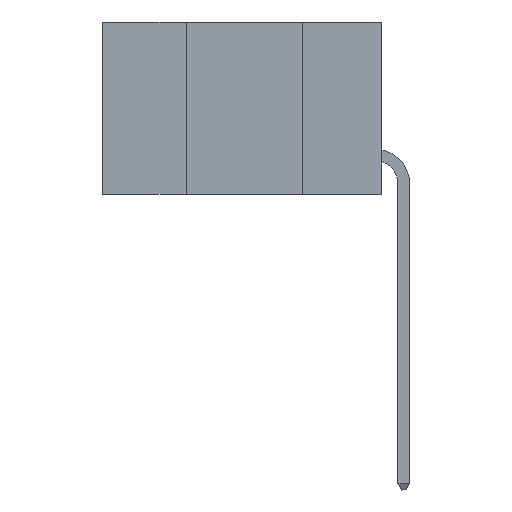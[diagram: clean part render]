
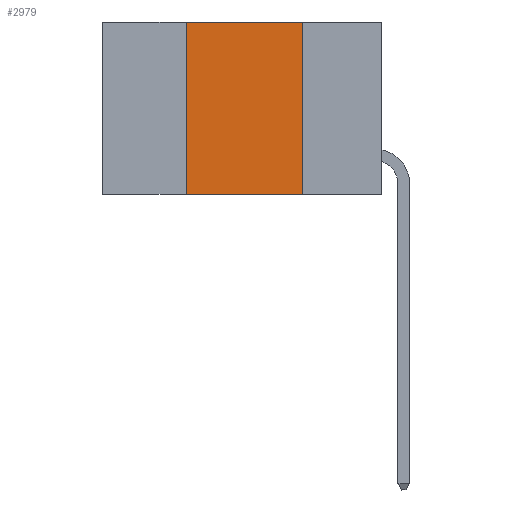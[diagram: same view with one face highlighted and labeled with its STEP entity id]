
A CAD part, left-side view. The second image highlights one B-rep face of the part: STEP entity #2979.
In plain terms, the highlighted planar face has unit normal (-1, 0, 0).
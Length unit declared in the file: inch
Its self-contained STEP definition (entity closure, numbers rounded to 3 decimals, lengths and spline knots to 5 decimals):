
#18 = LINE ( 'NONE', #8990, #13472 ) ;
#516 = DIRECTION ( 'NONE',  ( 0., 0., 1. ) ) ;
#536 = CARTESIAN_POINT ( 'NONE',  ( 0., 0.17, 0. ) ) ;
#847 = CARTESIAN_POINT ( 'NONE',  ( 0., 0.17, 0. ) ) ;
#995 = ORIENTED_EDGE ( 'NONE', *, *, #8402, .T. ) ;
#1134 = EDGE_CURVE ( 'NONE', #13733, #5274, #7700, .T. ) ;
#1401 = VECTOR ( 'NONE', #516, 39.37008 ) ;
#1699 = CARTESIAN_POINT ( 'NONE',  ( 0., 0.6, 0. ) ) ;
#1968 = EDGE_LOOP ( 'NONE', ( #12628, #9195, #4898, #995 ) ) ;
#2805 = DIRECTION ( 'NONE',  ( 0., -1., 0. ) ) ;
#2834 = PLANE ( 'NONE',  #4515 ) ;
#2979 = ADVANCED_FACE ( 'NONE', ( #12373 ), #2834, .F. ) ;
#3262 = EDGE_CURVE ( 'NONE', #5274, #13558, #8850, .T. ) ;
#4515 = AXIS2_PLACEMENT_3D ( 'NONE', #1699, #8485, #8434 ) ;
#4619 = CARTESIAN_POINT ( 'NONE',  ( 0., 0.17, -0.37 ) ) ;
#4898 = ORIENTED_EDGE ( 'NONE', *, *, #1134, .F. ) ;
#5102 = DIRECTION ( 'NONE',  ( 0., 0., -1. ) ) ;
#5274 = VERTEX_POINT ( 'NONE', #11314 ) ;
#5590 = VECTOR ( 'NONE', #5102, 39.37008 ) ;
#6688 = EDGE_CURVE ( 'NONE', #13558, #8736, #7886, .T. ) ;
#6861 = CARTESIAN_POINT ( 'NONE',  ( 0., 0.6, 0. ) ) ;
#7570 = CARTESIAN_POINT ( 'NONE',  ( 0., 0.42, -0.37 ) ) ;
#7700 = LINE ( 'NONE', #13897, #1401 ) ;
#7886 = LINE ( 'NONE', #536, #5590 ) ;
#8402 = EDGE_CURVE ( 'NONE', #13733, #8736, #18, .T. ) ;
#8434 = DIRECTION ( 'NONE',  ( 0., 0., -1. ) ) ;
#8485 = DIRECTION ( 'NONE',  ( 1., 0., 0. ) ) ;
#8736 = VERTEX_POINT ( 'NONE', #4619 ) ;
#8850 = LINE ( 'NONE', #6861, #9739 ) ;
#8990 = CARTESIAN_POINT ( 'NONE',  ( 0., 0.6, -0.37 ) ) ;
#9195 = ORIENTED_EDGE ( 'NONE', *, *, #3262, .F. ) ;
#9739 = VECTOR ( 'NONE', #10386, 39.37008 ) ;
#10386 = DIRECTION ( 'NONE',  ( 0., -1., 0. ) ) ;
#11314 = CARTESIAN_POINT ( 'NONE',  ( 0., 0.42, 0. ) ) ;
#12373 = FACE_OUTER_BOUND ( 'NONE', #1968, .T. ) ;
#12628 = ORIENTED_EDGE ( 'NONE', *, *, #6688, .F. ) ;
#13472 = VECTOR ( 'NONE', #2805, 39.37008 ) ;
#13558 = VERTEX_POINT ( 'NONE', #847 ) ;
#13733 = VERTEX_POINT ( 'NONE', #7570 ) ;
#13897 = CARTESIAN_POINT ( 'NONE',  ( 0., 0.42, 0. ) ) ;
